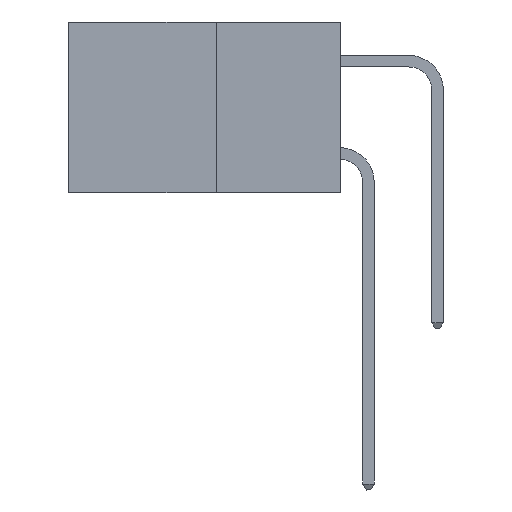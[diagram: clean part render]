
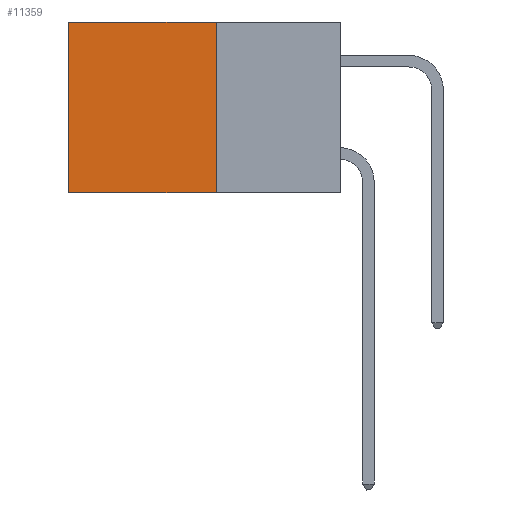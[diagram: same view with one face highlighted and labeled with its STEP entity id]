
A CAD part, left-side view. The second image highlights one B-rep face of the part: STEP entity #11359.
In plain terms, the highlighted planar face has unit normal (-1, 0, 0).
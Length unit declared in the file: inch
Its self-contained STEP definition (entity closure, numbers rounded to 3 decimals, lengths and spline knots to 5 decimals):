
#400 = VERTEX_POINT ( 'NONE', #6806 ) ;
#1370 = EDGE_CURVE ( 'NONE', #9741, #9846, #9062, .T. ) ;
#1925 = CARTESIAN_POINT ( 'NONE',  ( 0.277, 0.27, -0.37 ) ) ;
#2615 = EDGE_LOOP ( 'NONE', ( #8513, #10689, #7567, #7466 ) ) ;
#3203 = CARTESIAN_POINT ( 'NONE',  ( 0.277, 0.59, -0.37 ) ) ;
#3490 = FACE_OUTER_BOUND ( 'NONE', #2615, .T. ) ;
#3642 = LINE ( 'NONE', #15767, #4552 ) ;
#4185 = DIRECTION ( 'NONE',  ( 0., 1., 0. ) ) ;
#4552 = VECTOR ( 'NONE', #11547, 39.37008 ) ;
#4722 = VECTOR ( 'NONE', #8013, 39.37008 ) ;
#6806 = CARTESIAN_POINT ( 'NONE',  ( 0.277, 0.59, 0. ) ) ;
#7295 = DIRECTION ( 'NONE',  ( 0., 0., -1. ) ) ;
#7466 = ORIENTED_EDGE ( 'NONE', *, *, #13369, .T. ) ;
#7567 = ORIENTED_EDGE ( 'NONE', *, *, #11059, .F. ) ;
#7848 = PLANE ( 'NONE',  #10198 ) ;
#7908 = DIRECTION ( 'NONE',  ( 1., 0., 0. ) ) ;
#7969 = VECTOR ( 'NONE', #4185, 39.37008 ) ;
#8013 = DIRECTION ( 'NONE',  ( 0., 1., 0. ) ) ;
#8505 = CARTESIAN_POINT ( 'NONE',  ( 0.277, 0.27, 0. ) ) ;
#8513 = ORIENTED_EDGE ( 'NONE', *, *, #13423, .T. ) ;
#9062 = LINE ( 'NONE', #1925, #4722 ) ;
#9741 = VERTEX_POINT ( 'NONE', #9777 ) ;
#9777 = CARTESIAN_POINT ( 'NONE',  ( 0.277, 0.27, -0.37 ) ) ;
#9846 = VERTEX_POINT ( 'NONE', #3203 ) ;
#10198 = AXIS2_PLACEMENT_3D ( 'NONE', #15077, #7908, #17866 ) ;
#10689 = ORIENTED_EDGE ( 'NONE', *, *, #1370, .F. ) ;
#11059 = EDGE_CURVE ( 'NONE', #15539, #9741, #12148, .T. ) ;
#11359 = ADVANCED_FACE ( 'NONE', ( #3490 ), #7848, .F. ) ;
#11547 = DIRECTION ( 'NONE',  ( 0., 0., -1. ) ) ;
#12148 = LINE ( 'NONE', #15890, #15879 ) ;
#12310 = LINE ( 'NONE', #8505, #7969 ) ;
#13369 = EDGE_CURVE ( 'NONE', #15539, #400, #12310, .T. ) ;
#13423 = EDGE_CURVE ( 'NONE', #400, #9846, #3642, .T. ) ;
#15077 = CARTESIAN_POINT ( 'NONE',  ( 0.277, 0.27, -0.37 ) ) ;
#15539 = VERTEX_POINT ( 'NONE', #17398 ) ;
#15767 = CARTESIAN_POINT ( 'NONE',  ( 0.277, 0.59, -0.37 ) ) ;
#15879 = VECTOR ( 'NONE', #7295, 39.37008 ) ;
#15890 = CARTESIAN_POINT ( 'NONE',  ( 0.277, 0.27, -0.37 ) ) ;
#17398 = CARTESIAN_POINT ( 'NONE',  ( 0.277, 0.27, 0. ) ) ;
#17866 = DIRECTION ( 'NONE',  ( 0., 0., -1. ) ) ;
